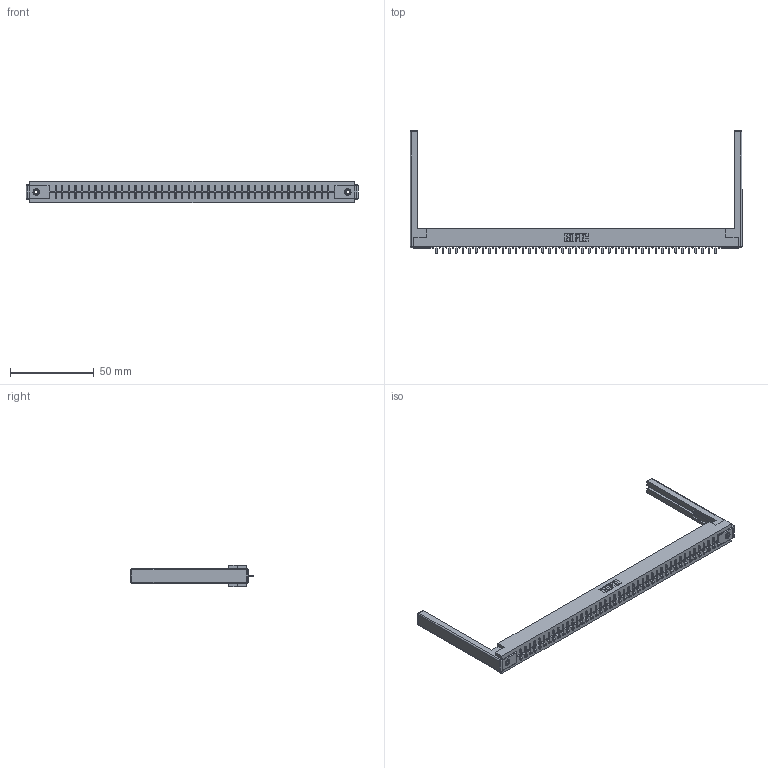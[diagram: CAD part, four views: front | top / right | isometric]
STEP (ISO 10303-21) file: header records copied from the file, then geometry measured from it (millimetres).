
FILE_DESCRIPTION (( 'STEP AP203' ), '1' );
FILE_NAME ('316-043-421-168.STEP', '2020-09-23T08:12:45', ( '' ), ( '' ), 'SwSTEP 2.0', 'SolidWorks 2020', '' );
FILE_SCHEMA (( 'CONFIG_CONTROL_DESIGN' ));
Length unit declared in the file: inch
Products named in the file (5): 306 Part_.156 Dia; 306-290-001_121; 307-220-068; 316-043-421-168; 345-250-001_345-250-001-102
Assembly tree (48 placements, depth 2):
  316-043-421-168
    306 Part_.156 Dia
    306-290-001_121  x43
    345-250-001_345-250-001-102  x2
    307-220-068  x2
Bounding box: 197.82 x 73.18 x 12.7 mm (x, y, z)
Volume: 26200.3 mm3; surface area: 26159.2 mm2
Topology: 48 solids, 48 shells, 3280 faces, 9177 edges, 5866 vertices
Faces by surface type: plane 2177, cylinder 907, sphere 180, cone 12, torus 4
Entity records: 42685 total; most frequent: CARTESIAN_POINT 7133, ORIENTED_EDGE 7064, DIRECTION 7046, EDGE_CURVE 3532, VECTOR 2760, LINE 2760, VERTEX_POINT 2230, AXIS2_PLACEMENT_3D 2143
